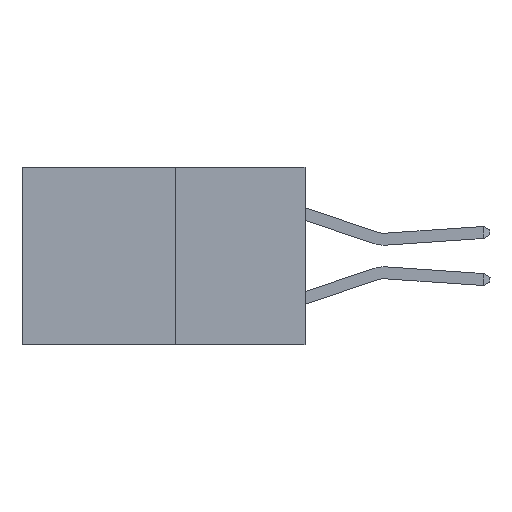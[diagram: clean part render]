
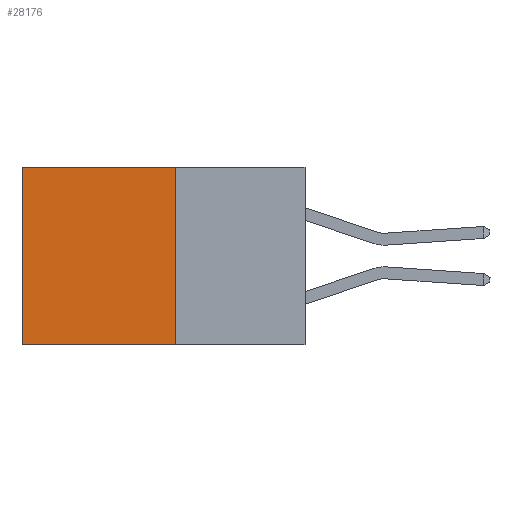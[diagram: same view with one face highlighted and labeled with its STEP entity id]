
A CAD part, left-side view. The second image highlights one B-rep face of the part: STEP entity #28176.
In plain terms, the highlighted planar face has unit normal (-1, 0, 0).
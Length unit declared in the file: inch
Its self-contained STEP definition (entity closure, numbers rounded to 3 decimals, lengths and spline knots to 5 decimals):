
#1898 = DIRECTION ( 'NONE',  ( 0., 0., -1. ) ) ;
#2377 = CARTESIAN_POINT ( 'NONE',  ( 0.277, 0.27, 0. ) ) ;
#2794 = VERTEX_POINT ( 'NONE', #13487 ) ;
#3697 = DIRECTION ( 'NONE',  ( 0., 1., 0. ) ) ;
#5012 = DIRECTION ( 'NONE',  ( 0., 0., -1. ) ) ;
#5896 = CARTESIAN_POINT ( 'NONE',  ( 0.277, 0.27, -0.37 ) ) ;
#6018 = LINE ( 'NONE', #5896, #31261 ) ;
#6335 = CARTESIAN_POINT ( 'NONE',  ( 0.277, 0.27, -0.37 ) ) ;
#7460 = LINE ( 'NONE', #19639, #25404 ) ;
#8046 = CARTESIAN_POINT ( 'NONE',  ( 0.277, 0.59, 0. ) ) ;
#8695 = LINE ( 'NONE', #31218, #27410 ) ;
#9971 = FACE_OUTER_BOUND ( 'NONE', #19035, .T. ) ;
#10224 = ORIENTED_EDGE ( 'NONE', *, *, #21927, .F. ) ;
#12079 = VECTOR ( 'NONE', #3697, 39.37008 ) ;
#12838 = LINE ( 'NONE', #20914, #12079 ) ;
#13487 = CARTESIAN_POINT ( 'NONE',  ( 0.277, 0.59, -0.37 ) ) ;
#14617 = CARTESIAN_POINT ( 'NONE',  ( 0.277, 0.27, -0.37 ) ) ;
#15248 = VERTEX_POINT ( 'NONE', #2377 ) ;
#15813 = EDGE_CURVE ( 'NONE', #21408, #2794, #8695, .T. ) ;
#17061 = DIRECTION ( 'NONE',  ( 0., 0., -1. ) ) ;
#18282 = AXIS2_PLACEMENT_3D ( 'NONE', #14617, #31712, #17061 ) ;
#19035 = EDGE_LOOP ( 'NONE', ( #27639, #20390, #10224, #24725 ) ) ;
#19639 = CARTESIAN_POINT ( 'NONE',  ( 0.277, 0.27, -0.37 ) ) ;
#20390 = ORIENTED_EDGE ( 'NONE', *, *, #29201, .F. ) ;
#20535 = DIRECTION ( 'NONE',  ( 0., 1., 0. ) ) ;
#20914 = CARTESIAN_POINT ( 'NONE',  ( 0.277, 0.27, 0. ) ) ;
#21408 = VERTEX_POINT ( 'NONE', #8046 ) ;
#21927 = EDGE_CURVE ( 'NONE', #15248, #23743, #7460, .T. ) ;
#23743 = VERTEX_POINT ( 'NONE', #6335 ) ;
#24725 = ORIENTED_EDGE ( 'NONE', *, *, #30976, .T. ) ;
#25404 = VECTOR ( 'NONE', #5012, 39.37008 ) ;
#27410 = VECTOR ( 'NONE', #1898, 39.37008 ) ;
#27639 = ORIENTED_EDGE ( 'NONE', *, *, #15813, .T. ) ;
#28176 = ADVANCED_FACE ( 'NONE', ( #9971 ), #29250, .F. ) ;
#29201 = EDGE_CURVE ( 'NONE', #23743, #2794, #6018, .T. ) ;
#29250 = PLANE ( 'NONE',  #18282 ) ;
#30976 = EDGE_CURVE ( 'NONE', #15248, #21408, #12838, .T. ) ;
#31218 = CARTESIAN_POINT ( 'NONE',  ( 0.277, 0.59, -0.37 ) ) ;
#31261 = VECTOR ( 'NONE', #20535, 39.37008 ) ;
#31712 = DIRECTION ( 'NONE',  ( 1., 0., 0. ) ) ;
